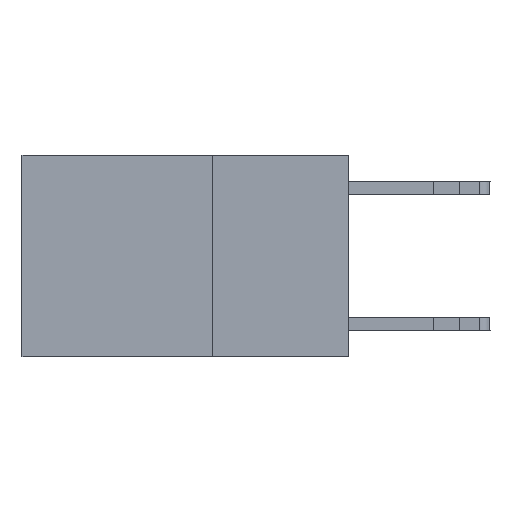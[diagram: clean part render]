
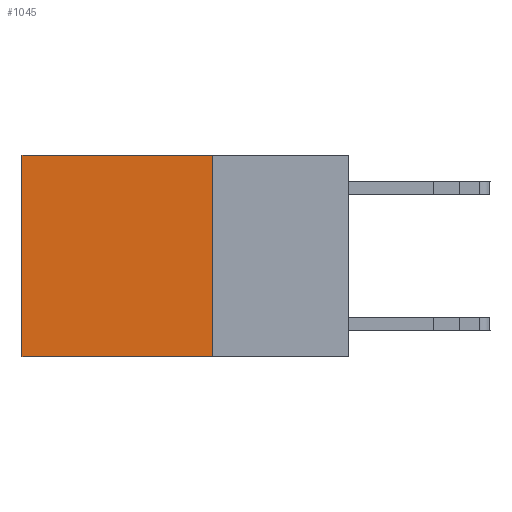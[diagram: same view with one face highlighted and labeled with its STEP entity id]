
A CAD part, left-side view. The second image highlights one B-rep face of the part: STEP entity #1045.
In plain terms, the highlighted planar face has unit normal (-1, 0, 0).
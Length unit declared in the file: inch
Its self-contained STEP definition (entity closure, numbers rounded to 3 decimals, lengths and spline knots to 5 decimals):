
#445 = VERTEX_POINT ( 'NONE', #7698 ) ;
#725 = ORIENTED_EDGE ( 'NONE', *, *, #1338, .F. ) ;
#954 = CARTESIAN_POINT ( 'NONE',  ( 0.2625, 0.25, 0. ) ) ;
#1045 = ADVANCED_FACE ( 'NONE', ( #12615 ), #17152, .F. ) ;
#1338 = EDGE_CURVE ( 'NONE', #18048, #445, #15815, .T. ) ;
#1783 = LINE ( 'NONE', #10782, #12289 ) ;
#1808 = VECTOR ( 'NONE', #13372, 39.37008 ) ;
#1810 = CARTESIAN_POINT ( 'NONE',  ( 0.2625, 0.25, 0. ) ) ;
#3351 = VECTOR ( 'NONE', #3741, 39.37008 ) ;
#3741 = DIRECTION ( 'NONE',  ( 0., 0., -1. ) ) ;
#4563 = VECTOR ( 'NONE', #9946, 39.37008 ) ;
#4647 = CARTESIAN_POINT ( 'NONE',  ( 0.2625, 0.6, 0. ) ) ;
#5483 = EDGE_CURVE ( 'NONE', #445, #6759, #13466, .T. ) ;
#6636 = EDGE_CURVE ( 'NONE', #18048, #15353, #1783, .T. ) ;
#6759 = VERTEX_POINT ( 'NONE', #19489 ) ;
#7253 = CARTESIAN_POINT ( 'NONE',  ( 0.2625, 0.6, 0. ) ) ;
#7311 = EDGE_LOOP ( 'NONE', ( #13165, #8772, #725, #7582 ) ) ;
#7582 = ORIENTED_EDGE ( 'NONE', *, *, #6636, .T. ) ;
#7698 = CARTESIAN_POINT ( 'NONE',  ( 0.2625, 0.25, -0.37 ) ) ;
#8772 = ORIENTED_EDGE ( 'NONE', *, *, #5483, .F. ) ;
#9487 = DIRECTION ( 'NONE',  ( 0., 0., -1. ) ) ;
#9946 = DIRECTION ( 'NONE',  ( 0., 1., 0. ) ) ;
#10782 = CARTESIAN_POINT ( 'NONE',  ( 0.2625, 0.25, 0. ) ) ;
#12289 = VECTOR ( 'NONE', #18527, 39.37008 ) ;
#12615 = FACE_OUTER_BOUND ( 'NONE', #7311, .T. ) ;
#12960 = AXIS2_PLACEMENT_3D ( 'NONE', #1810, #16948, #9487 ) ;
#13165 = ORIENTED_EDGE ( 'NONE', *, *, #13458, .T. ) ;
#13372 = DIRECTION ( 'NONE',  ( 0., 0., -1. ) ) ;
#13458 = EDGE_CURVE ( 'NONE', #15353, #6759, #19302, .T. ) ;
#13466 = LINE ( 'NONE', #19493, #4563 ) ;
#15353 = VERTEX_POINT ( 'NONE', #4647 ) ;
#15729 = CARTESIAN_POINT ( 'NONE',  ( 0.2625, 0.25, 0. ) ) ;
#15815 = LINE ( 'NONE', #954, #3351 ) ;
#16948 = DIRECTION ( 'NONE',  ( 1., 0., 0. ) ) ;
#17152 = PLANE ( 'NONE',  #12960 ) ;
#18048 = VERTEX_POINT ( 'NONE', #15729 ) ;
#18527 = DIRECTION ( 'NONE',  ( 0., 1., 0. ) ) ;
#19302 = LINE ( 'NONE', #7253, #1808 ) ;
#19489 = CARTESIAN_POINT ( 'NONE',  ( 0.2625, 0.6, -0.37 ) ) ;
#19493 = CARTESIAN_POINT ( 'NONE',  ( 0.2625, 0.25, -0.37 ) ) ;
